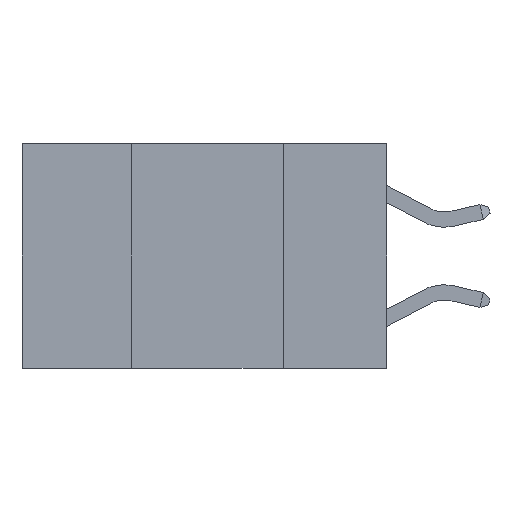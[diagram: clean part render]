
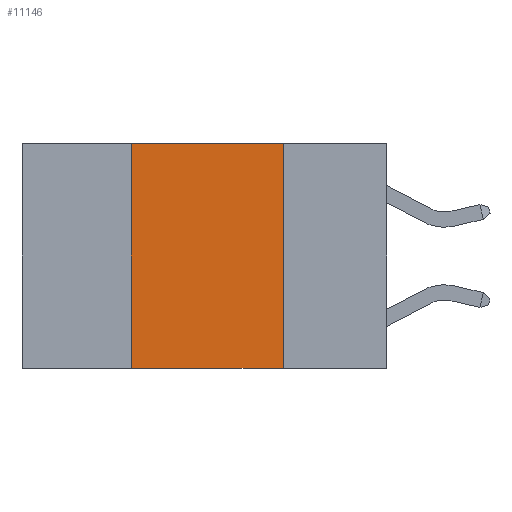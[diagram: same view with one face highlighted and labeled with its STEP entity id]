
A CAD part, left-side view. The second image highlights one B-rep face of the part: STEP entity #11146.
In plain terms, the highlighted planar face has unit normal (-1, 0, 0).
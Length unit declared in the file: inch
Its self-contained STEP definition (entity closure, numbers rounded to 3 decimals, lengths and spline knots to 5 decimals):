
#77 = DIRECTION ( 'NONE',  ( 0., 0., -1. ) ) ;
#202 = VERTEX_POINT ( 'NONE', #11600 ) ;
#248 = FACE_OUTER_BOUND ( 'NONE', #10369, .T. ) ;
#384 = LINE ( 'NONE', #4798, #9545 ) ;
#736 = AXIS2_PLACEMENT_3D ( 'NONE', #6148, #10692, #77 ) ;
#1363 = VERTEX_POINT ( 'NONE', #6414 ) ;
#1456 = ORIENTED_EDGE ( 'NONE', *, *, #12338, .F. ) ;
#1681 = VERTEX_POINT ( 'NONE', #5892 ) ;
#1821 = LINE ( 'NONE', #5653, #13717 ) ;
#2216 = CARTESIAN_POINT ( 'NONE',  ( 0., 0.6, 0. ) ) ;
#2369 = DIRECTION ( 'NONE',  ( 0., -1., 0. ) ) ;
#3108 = LINE ( 'NONE', #2216, #9040 ) ;
#4798 = CARTESIAN_POINT ( 'NONE',  ( 0., 0.17, 0. ) ) ;
#5653 = CARTESIAN_POINT ( 'NONE',  ( 0., 0.42, 0. ) ) ;
#5892 = CARTESIAN_POINT ( 'NONE',  ( 0., 0.17, -0.37 ) ) ;
#6010 = DIRECTION ( 'NONE',  ( 0., 0., -1. ) ) ;
#6148 = CARTESIAN_POINT ( 'NONE',  ( 0., 0.6, 0. ) ) ;
#6414 = CARTESIAN_POINT ( 'NONE',  ( 0., 0.42, 0. ) ) ;
#7303 = PLANE ( 'NONE',  #736 ) ;
#9040 = VECTOR ( 'NONE', #11630, 39.37008 ) ;
#9545 = VECTOR ( 'NONE', #6010, 39.37008 ) ;
#10213 = ORIENTED_EDGE ( 'NONE', *, *, #14939, .F. ) ;
#10235 = CARTESIAN_POINT ( 'NONE',  ( 0., 0.17, 0. ) ) ;
#10369 = EDGE_LOOP ( 'NONE', ( #10213, #10542, #1456, #10896 ) ) ;
#10542 = ORIENTED_EDGE ( 'NONE', *, *, #11692, .F. ) ;
#10692 = DIRECTION ( 'NONE',  ( 1., 0., 0. ) ) ;
#10896 = ORIENTED_EDGE ( 'NONE', *, *, #11750, .T. ) ;
#11146 = ADVANCED_FACE ( 'NONE', ( #248 ), #7303, .F. ) ;
#11378 = DIRECTION ( 'NONE',  ( 0., 0., 1. ) ) ;
#11600 = CARTESIAN_POINT ( 'NONE',  ( 0., 0.42, -0.37 ) ) ;
#11630 = DIRECTION ( 'NONE',  ( 0., -1., 0. ) ) ;
#11667 = LINE ( 'NONE', #13837, #14194 ) ;
#11692 = EDGE_CURVE ( 'NONE', #1363, #12885, #3108, .T. ) ;
#11750 = EDGE_CURVE ( 'NONE', #202, #1681, #11667, .T. ) ;
#12338 = EDGE_CURVE ( 'NONE', #202, #1363, #1821, .T. ) ;
#12885 = VERTEX_POINT ( 'NONE', #10235 ) ;
#13717 = VECTOR ( 'NONE', #11378, 39.37008 ) ;
#13837 = CARTESIAN_POINT ( 'NONE',  ( 0., 0.6, -0.37 ) ) ;
#14194 = VECTOR ( 'NONE', #2369, 39.37008 ) ;
#14939 = EDGE_CURVE ( 'NONE', #12885, #1681, #384, .T. ) ;
